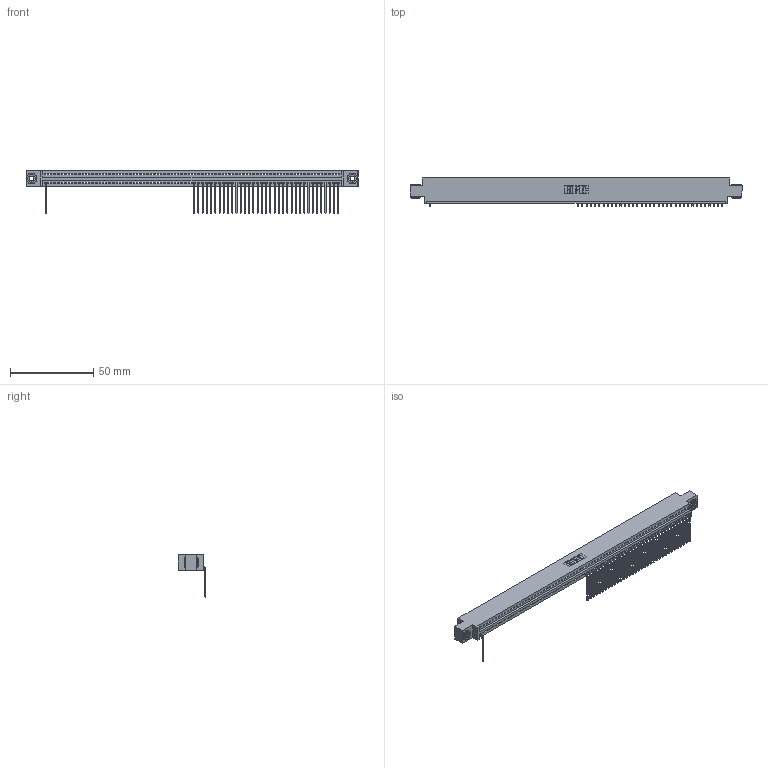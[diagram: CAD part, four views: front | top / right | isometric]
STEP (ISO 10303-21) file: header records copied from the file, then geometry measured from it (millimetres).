
FILE_DESCRIPTION (( 'STEP AP203' ), '1' );
FILE_NAME ('395-070-559-603.STEP', '2018-11-27T03:12:30', ( '' ), ( '' ), 'SwSTEP 2.0', 'SolidWorks 2016', '' );
FILE_SCHEMA (( 'CONFIG_CONTROL_DESIGN' ));
Length unit declared in the file: inch
Products named in the file (4): 345-250-002_345-250-002-102; 345-292-001_558 559 Tail - 1; 395-070-559-603; 345 Part_0.170 Offset - 0.156 Dia-TH
Assembly tree (39 placements, depth 2):
  395-070-559-603
    345 Part_0.170 Offset - 0.156 Dia-TH
    345-292-001_558 559 Tail - 1  x36
    345-250-002_345-250-002-102  x2
Bounding box: 199.01 x 16.75 x 25.53 mm (x, y, z)
Volume: 18768.1 mm3; surface area: 24299.9 mm2
Topology: 39 solids, 39 shells, 2872 faces, 8817 edges, 5826 vertices
Faces by surface type: plane 2082, cylinder 782, cone 8
Entity records: 48692 total; most frequent: ORIENTED_EDGE 8598, CARTESIAN_POINT 8567, DIRECTION 7433, EDGE_CURVE 4299, LINE 3863, VECTOR 3863, VERTEX_POINT 2862, AXIS2_PLACEMENT_3D 1785
